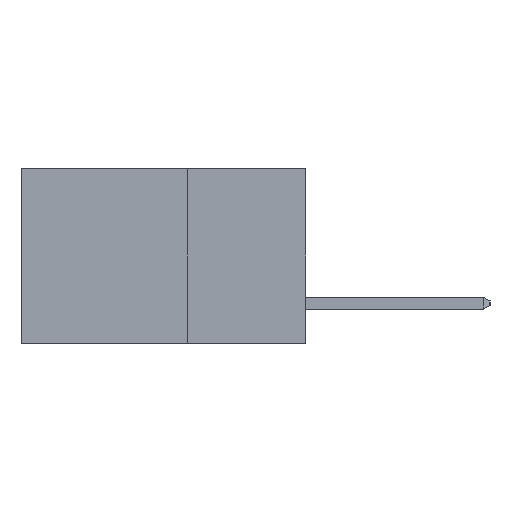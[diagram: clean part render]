
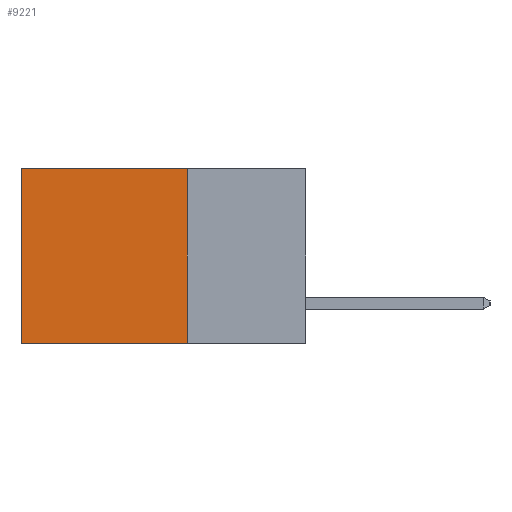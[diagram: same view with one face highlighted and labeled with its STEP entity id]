
A CAD part, left-side view. The second image highlights one B-rep face of the part: STEP entity #9221.
In plain terms, the highlighted planar face has unit normal (-1, 0, 0).
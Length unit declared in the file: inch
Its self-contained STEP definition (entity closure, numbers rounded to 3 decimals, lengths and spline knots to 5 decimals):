
#354 = ORIENTED_EDGE ( 'NONE', *, *, #4105, .F. ) ;
#690 = VECTOR ( 'NONE', #2898, 39.37008 ) ;
#1289 = VERTEX_POINT ( 'NONE', #3116 ) ;
#1386 = CARTESIAN_POINT ( 'NONE',  ( 0.298, 0.25, 0. ) ) ;
#1468 = LINE ( 'NONE', #5020, #10212 ) ;
#1971 = EDGE_LOOP ( 'NONE', ( #7494, #354, #1977, #2280 ) ) ;
#1977 = ORIENTED_EDGE ( 'NONE', *, *, #2160, .F. ) ;
#2160 = EDGE_CURVE ( 'NONE', #6511, #4514, #2985, .T. ) ;
#2256 = PLANE ( 'NONE',  #3096 ) ;
#2280 = ORIENTED_EDGE ( 'NONE', *, *, #10710, .T. ) ;
#2368 = FACE_OUTER_BOUND ( 'NONE', #1971, .T. ) ;
#2793 = CARTESIAN_POINT ( 'NONE',  ( 0.298, 0.25, 0. ) ) ;
#2898 = DIRECTION ( 'NONE',  ( 0., 0., -1. ) ) ;
#2985 = LINE ( 'NONE', #3199, #690 ) ;
#3096 = AXIS2_PLACEMENT_3D ( 'NONE', #1386, #3125, #9024 ) ;
#3116 = CARTESIAN_POINT ( 'NONE',  ( 0.298, 0.6, 0. ) ) ;
#3125 = DIRECTION ( 'NONE',  ( 1., 0., 0. ) ) ;
#3199 = CARTESIAN_POINT ( 'NONE',  ( 0.298, 0.25, 0. ) ) ;
#3599 = DIRECTION ( 'NONE',  ( 0., 1., 0. ) ) ;
#4105 = EDGE_CURVE ( 'NONE', #4514, #6773, #1468, .T. ) ;
#4209 = VECTOR ( 'NONE', #3599, 39.37008 ) ;
#4514 = VERTEX_POINT ( 'NONE', #4752 ) ;
#4576 = EDGE_CURVE ( 'NONE', #1289, #6773, #8754, .T. ) ;
#4752 = CARTESIAN_POINT ( 'NONE',  ( 0.298, 0.25, -0.37 ) ) ;
#5020 = CARTESIAN_POINT ( 'NONE',  ( 0.298, 0.25, -0.37 ) ) ;
#5369 = CARTESIAN_POINT ( 'NONE',  ( 0.298, 0.6, 0. ) ) ;
#6511 = VERTEX_POINT ( 'NONE', #10463 ) ;
#6773 = VERTEX_POINT ( 'NONE', #8489 ) ;
#7494 = ORIENTED_EDGE ( 'NONE', *, *, #4576, .T. ) ;
#8422 = LINE ( 'NONE', #2793, #4209 ) ;
#8489 = CARTESIAN_POINT ( 'NONE',  ( 0.298, 0.6, -0.37 ) ) ;
#8494 = VECTOR ( 'NONE', #10840, 39.37008 ) ;
#8754 = LINE ( 'NONE', #5369, #8494 ) ;
#9024 = DIRECTION ( 'NONE',  ( 0., 0., -1. ) ) ;
#9221 = ADVANCED_FACE ( 'NONE', ( #2368 ), #2256, .F. ) ;
#9892 = DIRECTION ( 'NONE',  ( 0., 1., 0. ) ) ;
#10212 = VECTOR ( 'NONE', #9892, 39.37008 ) ;
#10463 = CARTESIAN_POINT ( 'NONE',  ( 0.298, 0.25, 0. ) ) ;
#10710 = EDGE_CURVE ( 'NONE', #6511, #1289, #8422, .T. ) ;
#10840 = DIRECTION ( 'NONE',  ( 0., 0., -1. ) ) ;
